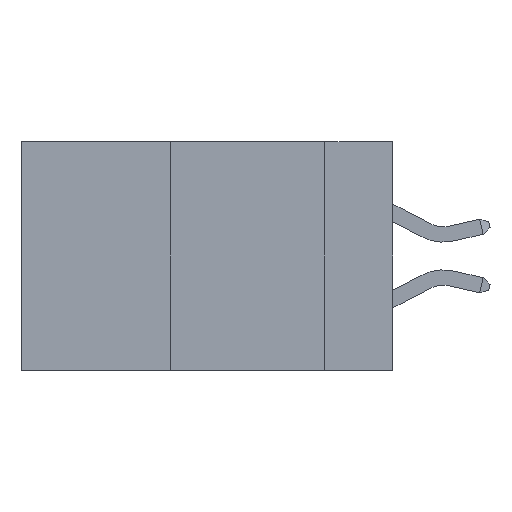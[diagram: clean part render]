
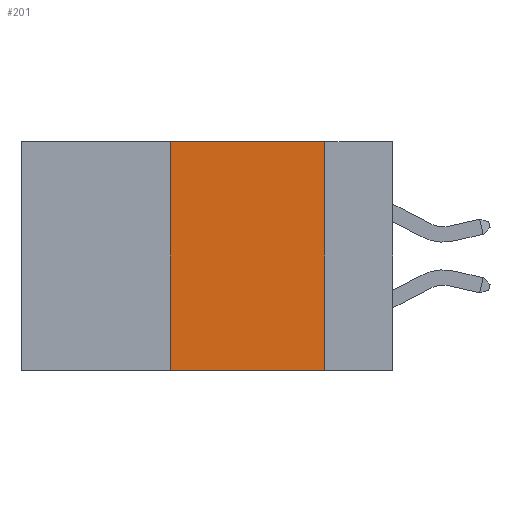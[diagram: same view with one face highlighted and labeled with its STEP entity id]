
A CAD part, left-side view. The second image highlights one B-rep face of the part: STEP entity #201.
In plain terms, the highlighted planar face has unit normal (-1, 0, 0).
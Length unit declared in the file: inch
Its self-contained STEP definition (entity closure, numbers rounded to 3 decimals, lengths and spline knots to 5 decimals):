
#201 = ADVANCED_FACE ( 'NONE', ( #10541 ), #11868, .F. ) ;
#373 = EDGE_LOOP ( 'NONE', ( #1850, #2814, #2366, #2142 ) ) ;
#623 = LINE ( 'NONE', #775, #1021 ) ;
#775 = CARTESIAN_POINT ( 'NONE',  ( 0., 0.36, 0. ) ) ;
#1021 = VECTOR ( 'NONE', #5835, 39.37008 ) ;
#1152 = CARTESIAN_POINT ( 'NONE',  ( 0., 0.6, 0. ) ) ;
#1241 = DIRECTION ( 'NONE',  ( 1., 0., 0. ) ) ;
#1493 = CARTESIAN_POINT ( 'NONE',  ( 0., 0.36, 0. ) ) ;
#1619 = DIRECTION ( 'NONE',  ( 0., -1., 0. ) ) ;
#1850 = ORIENTED_EDGE ( 'NONE', *, *, #7502, .F. ) ;
#2142 = ORIENTED_EDGE ( 'NONE', *, *, #4007, .T. ) ;
#2366 = ORIENTED_EDGE ( 'NONE', *, *, #10836, .F. ) ;
#2811 = VECTOR ( 'NONE', #1619, 39.37008 ) ;
#2814 = ORIENTED_EDGE ( 'NONE', *, *, #4298, .F. ) ;
#2884 = CARTESIAN_POINT ( 'NONE',  ( 0., 0.11, 0. ) ) ;
#3302 = VECTOR ( 'NONE', #4943, 39.37008 ) ;
#3749 = VERTEX_POINT ( 'NONE', #8512 ) ;
#4007 = EDGE_CURVE ( 'NONE', #3749, #5163, #5829, .T. ) ;
#4298 = EDGE_CURVE ( 'NONE', #11497, #6979, #5395, .T. ) ;
#4943 = DIRECTION ( 'NONE',  ( 0., -1., 0. ) ) ;
#5044 = CARTESIAN_POINT ( 'NONE',  ( 0., 0.6, -0.37 ) ) ;
#5163 = VERTEX_POINT ( 'NONE', #6978 ) ;
#5395 = LINE ( 'NONE', #1152, #2811 ) ;
#5795 = AXIS2_PLACEMENT_3D ( 'NONE', #9322, #1241, #7729 ) ;
#5829 = LINE ( 'NONE', #5044, #3302 ) ;
#5835 = DIRECTION ( 'NONE',  ( 0., 0., 1. ) ) ;
#6978 = CARTESIAN_POINT ( 'NONE',  ( 0., 0.11, -0.37 ) ) ;
#6979 = VERTEX_POINT ( 'NONE', #8109 ) ;
#7502 = EDGE_CURVE ( 'NONE', #6979, #5163, #10361, .T. ) ;
#7729 = DIRECTION ( 'NONE',  ( 0., 0., -1. ) ) ;
#8109 = CARTESIAN_POINT ( 'NONE',  ( 0., 0.11, 0. ) ) ;
#8512 = CARTESIAN_POINT ( 'NONE',  ( 0., 0.36, -0.37 ) ) ;
#9322 = CARTESIAN_POINT ( 'NONE',  ( 0., 0.6, 0. ) ) ;
#10361 = LINE ( 'NONE', #2884, #10627 ) ;
#10506 = DIRECTION ( 'NONE',  ( 0., 0., -1. ) ) ;
#10541 = FACE_OUTER_BOUND ( 'NONE', #373, .T. ) ;
#10627 = VECTOR ( 'NONE', #10506, 39.37008 ) ;
#10836 = EDGE_CURVE ( 'NONE', #3749, #11497, #623, .T. ) ;
#11497 = VERTEX_POINT ( 'NONE', #1493 ) ;
#11868 = PLANE ( 'NONE',  #5795 ) ;
